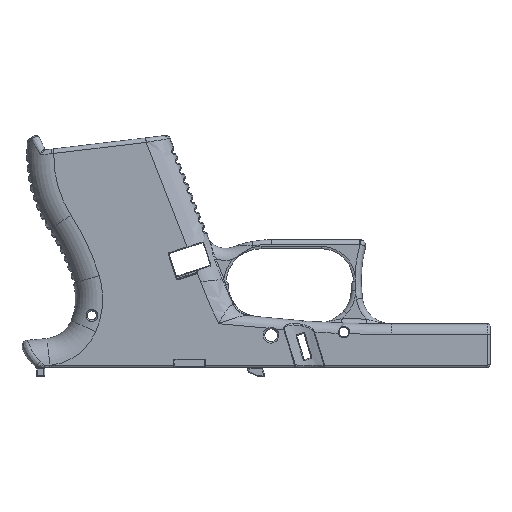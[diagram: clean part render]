
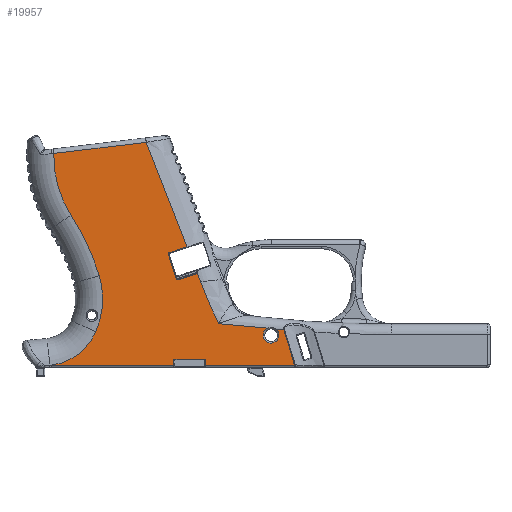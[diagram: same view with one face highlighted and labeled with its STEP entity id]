
A CAD part, front view. The second image highlights one B-rep face of the part: STEP entity #19957.
In plain terms, the highlighted planar face has unit normal (0, -1, 0).
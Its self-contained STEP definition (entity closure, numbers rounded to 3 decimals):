
#1344=CIRCLE('',#21159,27.167);
#1488=CIRCLE('',#21436,0.8);
#1493=CIRCLE('',#21449,2.625);
#1494=CIRCLE('',#21450,2.625);
#1495=CIRCLE('',#21451,156.771);
#1496=CIRCLE('',#21452,0.49);
#1497=CIRCLE('',#21453,0.49);
#1498=CIRCLE('',#21454,0.49);
#1499=CIRCLE('',#21455,35.645);
#1500=CIRCLE('',#21456,77.599);
#1501=CIRCLE('',#21457,18.891);
#3070=FACE_OUTER_BOUND('',#4384,.T.);
#4384=EDGE_LOOP('',(#13981,#13982,#13983,#13984,#13985,#13986,#13987,#13988,
#13989,#13990,#13991,#13992,#13993,#13994,#13995,#13996,#13997,#13998,#13999,
#14000,#14001,#14002,#14003,#14004,#14005,#14006,#14007,#14008));
#6160=LINE('',#32594,#7209);
#6161=LINE('',#32596,#7210);
#6162=LINE('',#32630,#7211);
#6170=LINE('',#32683,#7219);
#6171=LINE('',#32690,#7220);
#6172=LINE('',#32692,#7221);
#6173=LINE('',#32694,#7222);
#6174=LINE('',#32696,#7223);
#6175=LINE('',#32702,#7224);
#6176=LINE('',#32706,#7225);
#6177=LINE('',#32710,#7226);
#6178=LINE('',#32714,#7227);
#6179=LINE('',#32718,#7228);
#6180=LINE('',#32720,#7229);
#6181=LINE('',#32722,#7230);
#6182=LINE('',#32729,#7231);
#6183=LINE('',#32730,#7232);
#7209=VECTOR('',#24309,10.);
#7210=VECTOR('',#24312,10.);
#7211=VECTOR('',#24317,10.);
#7219=VECTOR('',#24345,10.);
#7220=VECTOR('',#24356,10.);
#7221=VECTOR('',#24357,10.);
#7222=VECTOR('',#24358,10.);
#7223=VECTOR('',#24359,10.);
#7224=VECTOR('',#24364,10.);
#7225=VECTOR('',#24367,10.);
#7226=VECTOR('',#24370,10.);
#7227=VECTOR('',#24373,10.);
#7228=VECTOR('',#24376,10.);
#7229=VECTOR('',#24377,10.);
#7230=VECTOR('',#24378,10.);
#7231=VECTOR('',#24385,10.);
#7232=VECTOR('',#24386,10.);
#8040=VERTEX_POINT('',#29518);
#8041=VERTEX_POINT('',#29520);
#8417=VERTEX_POINT('',#32245);
#8439=VERTEX_POINT('',#32414);
#8455=VERTEX_POINT('',#32592);
#8456=VERTEX_POINT('',#32621);
#8458=VERTEX_POINT('',#32659);
#8466=VERTEX_POINT('',#32681);
#8467=VERTEX_POINT('',#32689);
#8468=VERTEX_POINT('',#32691);
#8469=VERTEX_POINT('',#32693);
#8470=VERTEX_POINT('',#32695);
#8471=VERTEX_POINT('',#32697);
#8472=VERTEX_POINT('',#32699);
#8473=VERTEX_POINT('',#32701);
#8474=VERTEX_POINT('',#32703);
#8475=VERTEX_POINT('',#32705);
#8476=VERTEX_POINT('',#32707);
#8477=VERTEX_POINT('',#32709);
#8478=VERTEX_POINT('',#32711);
#8479=VERTEX_POINT('',#32713);
#8480=VERTEX_POINT('',#32715);
#8481=VERTEX_POINT('',#32717);
#8482=VERTEX_POINT('',#32719);
#8483=VERTEX_POINT('',#32721);
#8484=VERTEX_POINT('',#32723);
#8485=VERTEX_POINT('',#32726);
#8486=VERTEX_POINT('',#32728);
#9949=EDGE_CURVE('',#8040,#8041,#1344,.T.);
#10481=EDGE_CURVE('',#8455,#8417,#6160,.T.);
#10482=EDGE_CURVE('',#8417,#8439,#6161,.T.);
#10485=EDGE_CURVE('',#8439,#8456,#6162,.T.);
#10488=EDGE_CURVE('',#8456,#8458,#1488,.T.);
#10500=EDGE_CURVE('',#8466,#8455,#6170,.T.);
#10503=EDGE_CURVE('',#8467,#8466,#6171,.T.);
#10504=EDGE_CURVE('',#8468,#8467,#6172,.T.);
#10505=EDGE_CURVE('',#8469,#8468,#6173,.T.);
#10506=EDGE_CURVE('',#8470,#8469,#6174,.T.);
#10507=EDGE_CURVE('',#8471,#8470,#1493,.T.);
#10508=EDGE_CURVE('',#8472,#8471,#1494,.T.);
#10509=EDGE_CURVE('',#8473,#8472,#6175,.T.);
#10510=EDGE_CURVE('',#8474,#8473,#1495,.T.);
#10511=EDGE_CURVE('',#8474,#8475,#6176,.T.);
#10512=EDGE_CURVE('',#8476,#8475,#1496,.T.);
#10513=EDGE_CURVE('',#8477,#8476,#6177,.T.);
#10514=EDGE_CURVE('',#8478,#8477,#1497,.T.);
#10515=EDGE_CURVE('',#8479,#8478,#6178,.T.);
#10516=EDGE_CURVE('',#8480,#8479,#1498,.T.);
#10517=EDGE_CURVE('',#8481,#8480,#6179,.T.);
#10518=EDGE_CURVE('',#8481,#8482,#6180,.T.);
#10519=EDGE_CURVE('',#8483,#8482,#6181,.T.);
#10520=EDGE_CURVE('',#8484,#8483,#1499,.T.);
#10521=EDGE_CURVE('',#8041,#8484,#1500,.T.);
#10522=EDGE_CURVE('',#8485,#8040,#1501,.T.);
#10523=EDGE_CURVE('',#8486,#8485,#6182,.T.);
#10524=EDGE_CURVE('',#8458,#8486,#6183,.T.);
#13981=ORIENTED_EDGE('',*,*,#10481,.F.);
#13982=ORIENTED_EDGE('',*,*,#10500,.F.);
#13983=ORIENTED_EDGE('',*,*,#10503,.F.);
#13984=ORIENTED_EDGE('',*,*,#10504,.F.);
#13985=ORIENTED_EDGE('',*,*,#10505,.F.);
#13986=ORIENTED_EDGE('',*,*,#10506,.F.);
#13987=ORIENTED_EDGE('',*,*,#10507,.F.);
#13988=ORIENTED_EDGE('',*,*,#10508,.F.);
#13989=ORIENTED_EDGE('',*,*,#10509,.F.);
#13990=ORIENTED_EDGE('',*,*,#10510,.F.);
#13991=ORIENTED_EDGE('',*,*,#10511,.T.);
#13992=ORIENTED_EDGE('',*,*,#10512,.F.);
#13993=ORIENTED_EDGE('',*,*,#10513,.F.);
#13994=ORIENTED_EDGE('',*,*,#10514,.F.);
#13995=ORIENTED_EDGE('',*,*,#10515,.F.);
#13996=ORIENTED_EDGE('',*,*,#10516,.F.);
#13997=ORIENTED_EDGE('',*,*,#10517,.F.);
#13998=ORIENTED_EDGE('',*,*,#10518,.T.);
#13999=ORIENTED_EDGE('',*,*,#10519,.F.);
#14000=ORIENTED_EDGE('',*,*,#10520,.F.);
#14001=ORIENTED_EDGE('',*,*,#10521,.F.);
#14002=ORIENTED_EDGE('',*,*,#9949,.F.);
#14003=ORIENTED_EDGE('',*,*,#10522,.F.);
#14004=ORIENTED_EDGE('',*,*,#10523,.F.);
#14005=ORIENTED_EDGE('',*,*,#10524,.F.);
#14006=ORIENTED_EDGE('',*,*,#10488,.F.);
#14007=ORIENTED_EDGE('',*,*,#10485,.F.);
#14008=ORIENTED_EDGE('',*,*,#10482,.F.);
#19630=PLANE('',#21448);
#19957=ADVANCED_FACE('',(#3070),#19630,.F.);
#21159=AXIS2_PLACEMENT_3D('',#29521,#23535,#23536);
#21436=AXIS2_PLACEMENT_3D('',#32660,#24322,#24323);
#21448=AXIS2_PLACEMENT_3D('',#32688,#24354,#24355);
#21449=AXIS2_PLACEMENT_3D('',#32698,#24360,#24361);
#21450=AXIS2_PLACEMENT_3D('',#32700,#24362,#24363);
#21451=AXIS2_PLACEMENT_3D('',#32704,#24365,#24366);
#21452=AXIS2_PLACEMENT_3D('',#32708,#24368,#24369);
#21453=AXIS2_PLACEMENT_3D('',#32712,#24371,#24372);
#21454=AXIS2_PLACEMENT_3D('',#32716,#24374,#24375);
#21455=AXIS2_PLACEMENT_3D('',#32724,#24379,#24380);
#21456=AXIS2_PLACEMENT_3D('',#32725,#24381,#24382);
#21457=AXIS2_PLACEMENT_3D('',#32727,#24383,#24384);
#23535=DIRECTION('center_axis',(0.,-1.,0.));
#23536=DIRECTION('ref_axis',(0.998,0.,-0.06));
#24309=DIRECTION('',(0.,0.,1.));
#24312=DIRECTION('',(-1.,0.,0.));
#24317=DIRECTION('',(0.,0.,-1.));
#24322=DIRECTION('center_axis',(0.,-1.,0.));
#24323=DIRECTION('ref_axis',(-0.707,0.,0.707));
#24345=DIRECTION('',(-1.,0.,0.));
#24354=DIRECTION('center_axis',(0.,1.,0.));
#24355=DIRECTION('ref_axis',(1.,0.,0.));
#24356=DIRECTION('',(0.,0.,1.));
#24357=DIRECTION('',(-1.,0.,0.));
#24358=DIRECTION('',(0.292,0.,-0.956));
#24359=DIRECTION('',(0.996,0.,-0.092));
#24360=DIRECTION('center_axis',(0.,-1.,0.));
#24361=DIRECTION('ref_axis',(-1.,0.,0.));
#24362=DIRECTION('center_axis',(0.,-1.,0.));
#24363=DIRECTION('ref_axis',(-1.,0.,0.));
#24364=DIRECTION('',(0.996,0.,-0.092));
#24365=DIRECTION('center_axis',(0.,-1.,0.));
#24366=DIRECTION('ref_axis',(-0.937,0.,-0.35));
#24367=DIRECTION('',(-0.363,0.,0.932));
#24368=DIRECTION('center_axis',(0.,-1.,0.));
#24369=DIRECTION('ref_axis',(0.891,0.,-0.454));
#24370=DIRECTION('',(0.951,0.,0.309));
#24371=DIRECTION('center_axis',(0.,-1.,0.));
#24372=DIRECTION('ref_axis',(-0.454,0.,-0.891));
#24373=DIRECTION('',(0.309,0.,-0.951));
#24374=DIRECTION('center_axis',(0.,-1.,0.));
#24375=DIRECTION('ref_axis',(-0.891,0.,0.454));
#24376=DIRECTION('',(-0.951,0.,-0.309));
#24377=DIRECTION('',(-0.363,0.,0.932));
#24378=DIRECTION('',(0.993,0.,0.119));
#24379=DIRECTION('center_axis',(0.,1.,0.));
#24380=DIRECTION('ref_axis',(-0.961,0.,-0.276));
#24381=DIRECTION('center_axis',(0.,-1.,0.));
#24382=DIRECTION('ref_axis',(0.907,0.,0.421));
#24383=DIRECTION('center_axis',(0.,-1.,0.));
#24384=DIRECTION('ref_axis',(0.592,0.,-0.806));
#24385=DIRECTION('',(-1.,0.,0.));
#24386=DIRECTION('',(0.,0.,-1.));
#29518=CARTESIAN_POINT('',(-55.002,-11.5,-14.602));
#29520=CARTESIAN_POINT('',(-53.881,-11.5,4.09));
#29521=CARTESIAN_POINT('Origin',(-79.899,-11.5,-3.729));
#32245=CARTESIAN_POINT('',(-18.52,-11.5,-23.745));
#32414=CARTESIAN_POINT('',(-28.98,-11.5,-23.745));
#32592=CARTESIAN_POINT('',(-18.52,-11.5,-24.675));
#32594=CARTESIAN_POINT('',(-18.52,-11.5,-7.056));
#32596=CARTESIAN_POINT('',(-10.264,-11.5,-23.745));
#32621=CARTESIAN_POINT('',(-28.98,-11.5,-25.148));
#32630=CARTESIAN_POINT('',(-28.98,-11.5,-7.056));
#32659=CARTESIAN_POINT('',(-29.05,-11.5,-25.475));
#32660=CARTESIAN_POINT('Origin',(-28.25,-11.5,-25.475));
#32681=CARTESIAN_POINT('',(-18.45,-11.5,-24.675));
#32683=CARTESIAN_POINT('',(-10.264,-11.5,-24.675));
#32688=CARTESIAN_POINT('Origin',(-1.777,-11.5,10.863));
#32689=CARTESIAN_POINT('',(-18.45,-11.5,-25.75));
#32690=CARTESIAN_POINT('',(-18.45,-11.5,-7.818));
#32691=CARTESIAN_POINT('',(11.185,-11.5,-25.75));
#32692=CARTESIAN_POINT('',(37.236,-11.5,-25.75));
#32693=CARTESIAN_POINT('',(7.57,-11.5,-13.924));
#32694=CARTESIAN_POINT('',(5.553,-11.5,-7.328));
#32695=CARTESIAN_POINT('',(4.906,-11.5,-13.679));
#32696=CARTESIAN_POINT('',(4.861,-11.5,-13.675));
#32697=CARTESIAN_POINT('',(5.968,-11.5,-15.788));
#32698=CARTESIAN_POINT('Origin',(3.343,-11.5,-15.788));
#32699=CARTESIAN_POINT('',(2.19,-11.5,-13.43));
#32700=CARTESIAN_POINT('Origin',(3.343,-11.5,-15.788));
#32701=CARTESIAN_POINT('',(-14.141,-11.5,-11.929));
#32702=CARTESIAN_POINT('',(4.861,-11.5,-13.675));
#32703=CARTESIAN_POINT('',(-20.166,-11.5,2.06));
#32704=CARTESIAN_POINT('Origin',(126.663,-11.5,57.001));
#32705=CARTESIAN_POINT('',(-21.238,-11.5,4.813));
#32706=CARTESIAN_POINT('',(-37.545,-11.5,46.678));
#32707=CARTESIAN_POINT('',(-21.428,-11.5,4.698));
#32708=CARTESIAN_POINT('Origin',(-21.58,-11.5,5.164));
#32709=CARTESIAN_POINT('',(-27.61,-11.5,2.69));
#32710=CARTESIAN_POINT('',(-11.516,-11.5,7.919));
#32711=CARTESIAN_POINT('',(-28.228,-11.5,3.004));
#32712=CARTESIAN_POINT('Origin',(-27.762,-11.5,3.156));
#32713=CARTESIAN_POINT('',(-30.854,-11.5,11.088));
#32714=CARTESIAN_POINT('',(-28.236,-11.5,3.028));
#32715=CARTESIAN_POINT('',(-30.54,-11.5,11.706));
#32716=CARTESIAN_POINT('Origin',(-30.388,-11.5,11.24));
#32717=CARTESIAN_POINT('',(-24.666,-11.5,13.614));
#32718=CARTESIAN_POINT('',(-17.775,-11.5,15.853));
#32719=CARTESIAN_POINT('',(-38.228,-11.5,48.431));
#32720=CARTESIAN_POINT('',(-37.545,-11.5,46.678));
#32721=CARTESIAN_POINT('',(-68.991,-11.5,44.75));
#32722=CARTESIAN_POINT('',(-18.413,-11.5,50.802));
#32723=CARTESIAN_POINT('',(-63.213,-11.5,24.169));
#32724=CARTESIAN_POINT('Origin',(-33.363,-11.5,43.651));
#32725=CARTESIAN_POINT('Origin',(-128.196,-11.5,-18.243));
#32726=CARTESIAN_POINT('',(-69.695,-11.5,-25.75));
#32727=CARTESIAN_POINT('Origin',(-72.315,-11.5,-7.041));
#32728=CARTESIAN_POINT('',(-29.05,-11.5,-25.75));
#32729=CARTESIAN_POINT('',(37.236,-11.5,-25.75));
#32730=CARTESIAN_POINT('',(-29.05,-11.5,-7.056));
